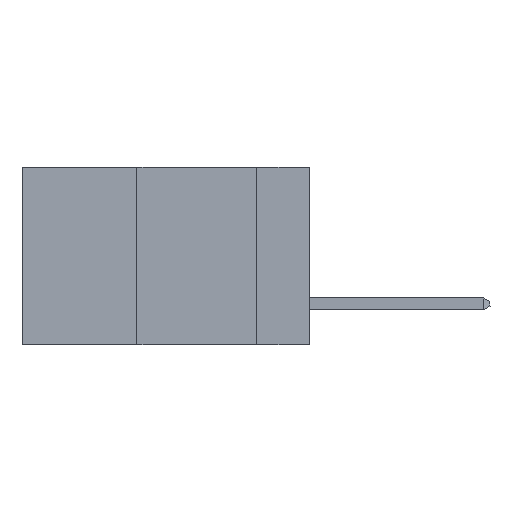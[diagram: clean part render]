
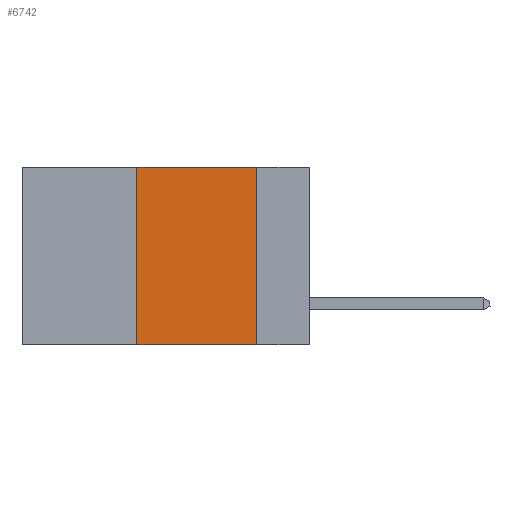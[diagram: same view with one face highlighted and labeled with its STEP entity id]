
A CAD part, left-side view. The second image highlights one B-rep face of the part: STEP entity #6742.
In plain terms, the highlighted planar face has unit normal (-1, 0, 0).
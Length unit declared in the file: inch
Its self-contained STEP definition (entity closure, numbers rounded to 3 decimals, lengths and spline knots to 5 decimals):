
#106 = ORIENTED_EDGE ( 'NONE', *, *, #8038, .F. ) ;
#289 = ORIENTED_EDGE ( 'NONE', *, *, #6227, .F. ) ;
#437 = VECTOR ( 'NONE', #2177, 39.37008 ) ;
#991 = PLANE ( 'NONE',  #3446 ) ;
#1102 = EDGE_LOOP ( 'NONE', ( #289, #5418, #106, #6521 ) ) ;
#1579 = DIRECTION ( 'NONE',  ( 0., -1., 0. ) ) ;
#1715 = DIRECTION ( 'NONE',  ( 0., 0., -1. ) ) ;
#1815 = CARTESIAN_POINT ( 'NONE',  ( 0., 0.36, 0. ) ) ;
#2177 = DIRECTION ( 'NONE',  ( 0., -1., 0. ) ) ;
#2494 = EDGE_CURVE ( 'NONE', #6563, #3068, #6752, .T. ) ;
#2583 = LINE ( 'NONE', #5519, #437 ) ;
#2795 = VECTOR ( 'NONE', #1579, 39.37008 ) ;
#2883 = VECTOR ( 'NONE', #8203, 39.37008 ) ;
#3002 = CARTESIAN_POINT ( 'NONE',  ( 0., 0.6, -0.37 ) ) ;
#3068 = VERTEX_POINT ( 'NONE', #6388 ) ;
#3216 = DIRECTION ( 'NONE',  ( 0., 0., -1. ) ) ;
#3446 = AXIS2_PLACEMENT_3D ( 'NONE', #5083, #5761, #1715 ) ;
#3534 = CARTESIAN_POINT ( 'NONE',  ( 0., 0.36, 0. ) ) ;
#3575 = VECTOR ( 'NONE', #3216, 39.37008 ) ;
#3672 = CARTESIAN_POINT ( 'NONE',  ( 0., 0.11, 0. ) ) ;
#4237 = CARTESIAN_POINT ( 'NONE',  ( 0., 0.36, -0.37 ) ) ;
#4278 = FACE_OUTER_BOUND ( 'NONE', #1102, .T. ) ;
#5083 = CARTESIAN_POINT ( 'NONE',  ( 0., 0.6, 0. ) ) ;
#5418 = ORIENTED_EDGE ( 'NONE', *, *, #6552, .F. ) ;
#5519 = CARTESIAN_POINT ( 'NONE',  ( 0., 0.6, 0. ) ) ;
#5761 = DIRECTION ( 'NONE',  ( 1., 0., 0. ) ) ;
#6227 = EDGE_CURVE ( 'NONE', #8185, #3068, #7074, .T. ) ;
#6388 = CARTESIAN_POINT ( 'NONE',  ( 0., 0.11, -0.37 ) ) ;
#6521 = ORIENTED_EDGE ( 'NONE', *, *, #2494, .T. ) ;
#6552 = EDGE_CURVE ( 'NONE', #7510, #8185, #2583, .T. ) ;
#6563 = VERTEX_POINT ( 'NONE', #4237 ) ;
#6742 = ADVANCED_FACE ( 'NONE', ( #4278 ), #991, .F. ) ;
#6752 = LINE ( 'NONE', #3002, #2795 ) ;
#7074 = LINE ( 'NONE', #7184, #3575 ) ;
#7184 = CARTESIAN_POINT ( 'NONE',  ( 0., 0.11, 0. ) ) ;
#7510 = VERTEX_POINT ( 'NONE', #1815 ) ;
#7779 = LINE ( 'NONE', #3534, #2883 ) ;
#8038 = EDGE_CURVE ( 'NONE', #6563, #7510, #7779, .T. ) ;
#8185 = VERTEX_POINT ( 'NONE', #3672 ) ;
#8203 = DIRECTION ( 'NONE',  ( 0., 0., 1. ) ) ;
